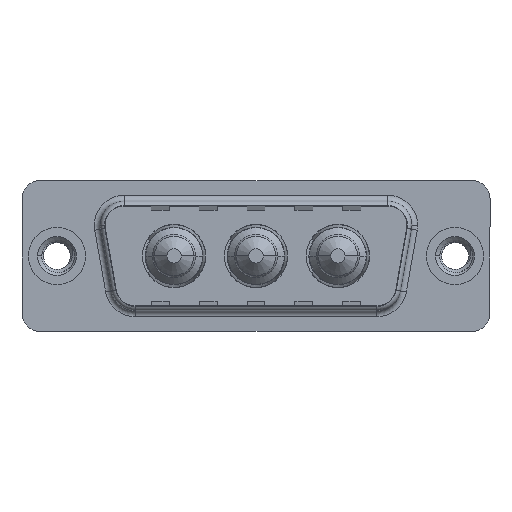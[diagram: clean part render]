
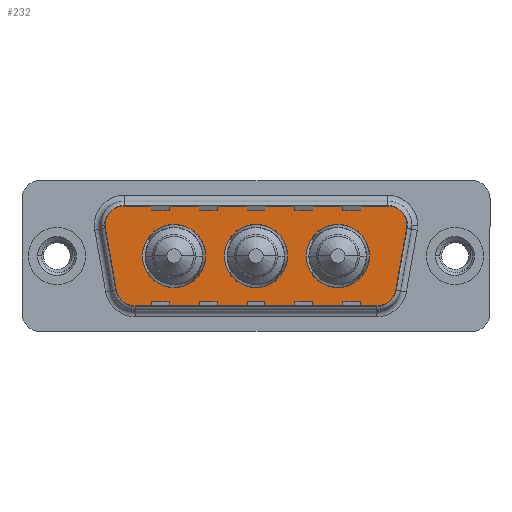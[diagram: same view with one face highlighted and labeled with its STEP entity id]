
A CAD part, top view. The second image highlights one B-rep face of the part: STEP entity #232.
In plain terms, the highlighted planar face has unit normal (0, 0, 1).
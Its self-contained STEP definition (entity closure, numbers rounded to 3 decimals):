
#45 = DIRECTION ( 'NONE',  ( 0., 0., 1. ) ) ;
#125 = DIRECTION ( 'NONE',  ( 0., 0., 1. ) ) ;
#232 = ADVANCED_FACE ( 'NONE', ( #7618, #2305, #7322, #4646 ), #697, .T. ) ;
#355 = DIRECTION ( 'NONE',  ( 0., 0., 1. ) ) ;
#356 = CARTESIAN_POINT ( 'NONE',  ( 26.866, -4.9, 0. ) ) ;
#376 = CIRCLE ( 'NONE', #10863, 2. ) ;
#434 = CARTESIAN_POINT ( 'NONE',  ( 5.411, 4.9, 0. ) ) ;
#506 = VERTEX_POINT ( 'NONE', #3483 ) ;
#697 = PLANE ( 'NONE',  #6273 ) ;
#755 = DIRECTION ( 'NONE',  ( 1., 0., 0. ) ) ;
#769 = DIRECTION ( 'NONE',  ( 0., 0., 1. ) ) ;
#776 = VERTEX_POINT ( 'NONE', #356 ) ;
#881 = CARTESIAN_POINT ( 'NONE',  ( 5.411, 2.9, 0. ) ) ;
#929 = VERTEX_POINT ( 'NONE', #3899 ) ;
#939 = ORIENTED_EDGE ( 'NONE', *, *, #8453, .T. ) ;
#1228 = DIRECTION ( 'NONE',  ( 1., 0., 0. ) ) ;
#1301 = CARTESIAN_POINT ( 'NONE',  ( 16.65, 0., 0. ) ) ;
#1327 = ORIENTED_EDGE ( 'NONE', *, *, #1529, .T. ) ;
#1408 = CIRCLE ( 'NONE', #4675, 2.65 ) ;
#1529 = EDGE_CURVE ( 'NONE', #8891, #9048, #4177, .T. ) ;
#1700 = CARTESIAN_POINT ( 'NONE',  ( 19.3, 0., 0. ) ) ;
#2045 = CARTESIAN_POINT ( 'NONE',  ( 16.65, 0., 0. ) ) ;
#2076 = CARTESIAN_POINT ( 'NONE',  ( 9.8, 0., 0. ) ) ;
#2152 = CIRCLE ( 'NONE', #7250, 2.65 ) ;
#2168 = DIRECTION ( 'NONE',  ( -1., 0., 0. ) ) ;
#2188 = DIRECTION ( 'NONE',  ( 0., 0., 1. ) ) ;
#2257 = ORIENTED_EDGE ( 'NONE', *, *, #3319, .T. ) ;
#2305 = FACE_BOUND ( 'NONE', #12051, .T. ) ;
#2464 = CARTESIAN_POINT ( 'NONE',  ( 4.464, -3.247, 0. ) ) ;
#2520 = AXIS2_PLACEMENT_3D ( 'NONE', #1301, #7805, #10683 ) ;
#2551 = CIRCLE ( 'NONE', #8344, 2.65 ) ;
#2654 = AXIS2_PLACEMENT_3D ( 'NONE', #881, #2858, #5071 ) ;
#2718 = EDGE_CURVE ( 'NONE', #9048, #9837, #4603, .T. ) ;
#2745 = ORIENTED_EDGE ( 'NONE', *, *, #2718, .T. ) ;
#2767 = AXIS2_PLACEMENT_3D ( 'NONE', #5221, #769, #755 ) ;
#2843 = EDGE_CURVE ( 'NONE', #8212, #5845, #3705, .T. ) ;
#2858 = DIRECTION ( 'NONE',  ( 0., 0., 1. ) ) ;
#2908 = LINE ( 'NONE', #12296, #4907 ) ;
#2967 = CIRCLE ( 'NONE', #3037, 2. ) ;
#3012 = CARTESIAN_POINT ( 'NONE',  ( 28.836, -3.247, 0. ) ) ;
#3037 = AXIS2_PLACEMENT_3D ( 'NONE', #8430, #125, #9563 ) ;
#3101 = DIRECTION ( 'NONE',  ( 1., 0., 0. ) ) ;
#3184 = ORIENTED_EDGE ( 'NONE', *, *, #8481, .T. ) ;
#3196 = CARTESIAN_POINT ( 'NONE',  ( 14., 0., 0. ) ) ;
#3208 = DIRECTION ( 'NONE',  ( -1., 0., 0. ) ) ;
#3238 = DIRECTION ( 'NONE',  ( 1., 0., 0. ) ) ;
#3319 = EDGE_CURVE ( 'NONE', #9837, #11514, #2908, .T. ) ;
#3397 = CARTESIAN_POINT ( 'NONE',  ( 12.45, 0., 0. ) ) ;
#3452 = DIRECTION ( 'NONE',  ( 0., 0., 1. ) ) ;
#3483 = CARTESIAN_POINT ( 'NONE',  ( 6.434, -4.9, 0. ) ) ;
#3514 = VECTOR ( 'NONE', #3238, 1000. ) ;
#3580 = ORIENTED_EDGE ( 'NONE', *, *, #10140, .F. ) ;
#3616 = ORIENTED_EDGE ( 'NONE', *, *, #2843, .F. ) ;
#3705 = CIRCLE ( 'NONE', #2520, 2.65 ) ;
#3785 = CARTESIAN_POINT ( 'NONE',  ( 23.5, 0., 0. ) ) ;
#3899 = CARTESIAN_POINT ( 'NONE',  ( 26.15, 0., 0. ) ) ;
#3916 = DIRECTION ( 'NONE',  ( -1., 0., 0. ) ) ;
#3920 = DIRECTION ( 'NONE',  ( 0., 0., 1. ) ) ;
#3927 = ORIENTED_EDGE ( 'NONE', *, *, #11927, .F. ) ;
#4117 = DIRECTION ( 'NONE',  ( 0.174, -0.985, 0. ) ) ;
#4177 = LINE ( 'NONE', #434, #8819 ) ;
#4312 = EDGE_CURVE ( 'NONE', #11325, #10425, #8012, .T. ) ;
#4391 = CARTESIAN_POINT ( 'NONE',  ( 9.8, 0., 0. ) ) ;
#4552 = LINE ( 'NONE', #10525, #7238 ) ;
#4553 = CARTESIAN_POINT ( 'NONE',  ( 26.866, -2.9, 0. ) ) ;
#4603 = CIRCLE ( 'NONE', #2654, 2. ) ;
#4646 = FACE_OUTER_BOUND ( 'NONE', #8509, .T. ) ;
#4647 = CARTESIAN_POINT ( 'NONE',  ( 27.889, 2.9, 0. ) ) ;
#4675 = AXIS2_PLACEMENT_3D ( 'NONE', #3785, #355, #9677 ) ;
#4830 = VERTEX_POINT ( 'NONE', #10813 ) ;
#4907 = VECTOR ( 'NONE', #4117, 1000. ) ;
#5071 = DIRECTION ( 'NONE',  ( 1., 0., 0. ) ) ;
#5221 = CARTESIAN_POINT ( 'NONE',  ( 26.866, -2.9, 0. ) ) ;
#5347 = EDGE_CURVE ( 'NONE', #506, #776, #11739, .T. ) ;
#5437 = DIRECTION ( 'NONE',  ( 1., 0., 0. ) ) ;
#5608 = CARTESIAN_POINT ( 'NONE',  ( 27.889, 2.9, 0. ) ) ;
#5787 = ORIENTED_EDGE ( 'NONE', *, *, #12540, .F. ) ;
#5845 = VERTEX_POINT ( 'NONE', #3196 ) ;
#5860 = ORIENTED_EDGE ( 'NONE', *, *, #5978, .F. ) ;
#5978 = EDGE_CURVE ( 'NONE', #4830, #929, #1408, .T. ) ;
#6015 = CARTESIAN_POINT ( 'NONE',  ( 5.411, 4.9, 0. ) ) ;
#6129 = EDGE_CURVE ( 'NONE', #9482, #11325, #4552, .T. ) ;
#6273 = AXIS2_PLACEMENT_3D ( 'NONE', #4553, #12963, #12251 ) ;
#6402 = EDGE_LOOP ( 'NONE', ( #8066, #5787 ) ) ;
#6416 = CIRCLE ( 'NONE', #9688, 2.65 ) ;
#6672 = VERTEX_POINT ( 'NONE', #12241 ) ;
#7238 = VECTOR ( 'NONE', #11464, 1000. ) ;
#7250 = AXIS2_PLACEMENT_3D ( 'NONE', #4391, #11378, #5437 ) ;
#7301 = AXIS2_PLACEMENT_3D ( 'NONE', #5608, #45, #2168 ) ;
#7322 = FACE_BOUND ( 'NONE', #6402, .T. ) ;
#7618 = FACE_BOUND ( 'NONE', #10171, .T. ) ;
#7805 = DIRECTION ( 'NONE',  ( 0., 0., 1. ) ) ;
#8012 = CIRCLE ( 'NONE', #7301, 2. ) ;
#8066 = ORIENTED_EDGE ( 'NONE', *, *, #8398, .F. ) ;
#8123 = CARTESIAN_POINT ( 'NONE',  ( 6.434, -4.9, 0. ) ) ;
#8212 = VERTEX_POINT ( 'NONE', #1700 ) ;
#8224 = EDGE_CURVE ( 'NONE', #11514, #506, #2967, .T. ) ;
#8344 = AXIS2_PLACEMENT_3D ( 'NONE', #9400, #3452, #10407 ) ;
#8398 = EDGE_CURVE ( 'NONE', #12095, #6672, #6416, .T. ) ;
#8430 = CARTESIAN_POINT ( 'NONE',  ( 6.434, -2.9, 0. ) ) ;
#8453 = EDGE_CURVE ( 'NONE', #10425, #8891, #376, .T. ) ;
#8481 = EDGE_CURVE ( 'NONE', #776, #9482, #10146, .T. ) ;
#8509 = EDGE_LOOP ( 'NONE', ( #3184, #10265, #10186, #939, #1327, #2745, #2257, #10300, #9179 ) ) ;
#8819 = VECTOR ( 'NONE', #3208, 1000. ) ;
#8891 = VERTEX_POINT ( 'NONE', #12215 ) ;
#9027 = DIRECTION ( 'NONE',  ( 0., 0., 1. ) ) ;
#9048 = VERTEX_POINT ( 'NONE', #6015 ) ;
#9179 = ORIENTED_EDGE ( 'NONE', *, *, #5347, .T. ) ;
#9400 = CARTESIAN_POINT ( 'NONE',  ( 23.5, 0., 0. ) ) ;
#9482 = VERTEX_POINT ( 'NONE', #3012 ) ;
#9563 = DIRECTION ( 'NONE',  ( -1., 0., 0. ) ) ;
#9677 = DIRECTION ( 'NONE',  ( 1., 0., 0. ) ) ;
#9688 = AXIS2_PLACEMENT_3D ( 'NONE', #2076, #3920, #1228 ) ;
#9741 = CARTESIAN_POINT ( 'NONE',  ( 29.889, 2.9, 0. ) ) ;
#9837 = VERTEX_POINT ( 'NONE', #11835 ) ;
#10017 = CIRCLE ( 'NONE', #11316, 2.65 ) ;
#10085 = CARTESIAN_POINT ( 'NONE',  ( 29.859, 2.553, 0. ) ) ;
#10140 = EDGE_CURVE ( 'NONE', #929, #4830, #2551, .T. ) ;
#10146 = CIRCLE ( 'NONE', #2767, 2. ) ;
#10171 = EDGE_LOOP ( 'NONE', ( #3616, #3927 ) ) ;
#10186 = ORIENTED_EDGE ( 'NONE', *, *, #4312, .T. ) ;
#10265 = ORIENTED_EDGE ( 'NONE', *, *, #6129, .T. ) ;
#10300 = ORIENTED_EDGE ( 'NONE', *, *, #8224, .T. ) ;
#10407 = DIRECTION ( 'NONE',  ( 1., 0., 0. ) ) ;
#10425 = VERTEX_POINT ( 'NONE', #9741 ) ;
#10525 = CARTESIAN_POINT ( 'NONE',  ( 29.859, 2.553, 0. ) ) ;
#10683 = DIRECTION ( 'NONE',  ( 1., 0., 0. ) ) ;
#10813 = CARTESIAN_POINT ( 'NONE',  ( 20.85, 0., 0. ) ) ;
#10863 = AXIS2_PLACEMENT_3D ( 'NONE', #4647, #2188, #3916 ) ;
#11316 = AXIS2_PLACEMENT_3D ( 'NONE', #2045, #9027, #3101 ) ;
#11325 = VERTEX_POINT ( 'NONE', #10085 ) ;
#11378 = DIRECTION ( 'NONE',  ( 0., 0., 1. ) ) ;
#11464 = DIRECTION ( 'NONE',  ( 0.174, 0.985, 0. ) ) ;
#11514 = VERTEX_POINT ( 'NONE', #2464 ) ;
#11739 = LINE ( 'NONE', #8123, #3514 ) ;
#11835 = CARTESIAN_POINT ( 'NONE',  ( 3.441, 2.553, 0. ) ) ;
#11927 = EDGE_CURVE ( 'NONE', #5845, #8212, #10017, .T. ) ;
#12051 = EDGE_LOOP ( 'NONE', ( #3580, #5860 ) ) ;
#12095 = VERTEX_POINT ( 'NONE', #3397 ) ;
#12215 = CARTESIAN_POINT ( 'NONE',  ( 27.889, 4.9, 0. ) ) ;
#12241 = CARTESIAN_POINT ( 'NONE',  ( 7.15, 0., 0. ) ) ;
#12251 = DIRECTION ( 'NONE',  ( 1., 0., 0. ) ) ;
#12296 = CARTESIAN_POINT ( 'NONE',  ( 3.441, 2.553, 0. ) ) ;
#12540 = EDGE_CURVE ( 'NONE', #6672, #12095, #2152, .T. ) ;
#12963 = DIRECTION ( 'NONE',  ( 0., 0., 1. ) ) ;
